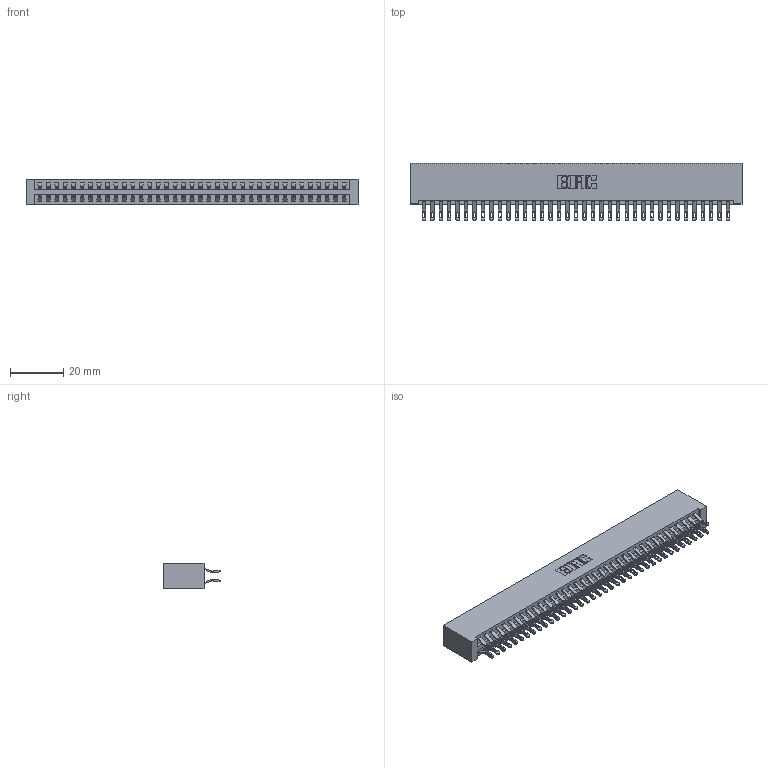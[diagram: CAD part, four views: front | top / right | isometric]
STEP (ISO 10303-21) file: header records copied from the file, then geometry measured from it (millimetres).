
FILE_DESCRIPTION (( 'STEP AP203' ), '1' );
FILE_NAME ('346-074-555-201.STEP', '2018-08-29T02:40:24', ( '' ), ( '' ), 'SwSTEP 2.0', 'SolidWorks 2016', '' );
FILE_SCHEMA (( 'CONFIG_CONTROL_DESIGN' ));
Length unit declared in the file: inch
Products named in the file (3): 346 Part_No Mounting Lugs; 345-292-001_555 Tail; 346-074-555-201
Assembly tree (75 placements, depth 2):
  346-074-555-201
    346 Part_No Mounting Lugs
    345-292-001_555 Tail  x74
Bounding box: 124.71 x 21.46 x 9.4 mm (x, y, z)
Volume: 12910.3 mm3; surface area: 18595.7 mm2
Topology: 75 solids, 75 shells, 4406 faces, 13847 edges, 9230 vertices
Faces by surface type: plane 2514, cylinder 1892
Entity records: 24869 total; most frequent: CARTESIAN_POINT 4138, ORIENTED_EDGE 4042, DIRECTION 3661, EDGE_CURVE 2021, LINE 1729, VECTOR 1729, VERTEX_POINT 1346, AXIS2_PLACEMENT_3D 966
